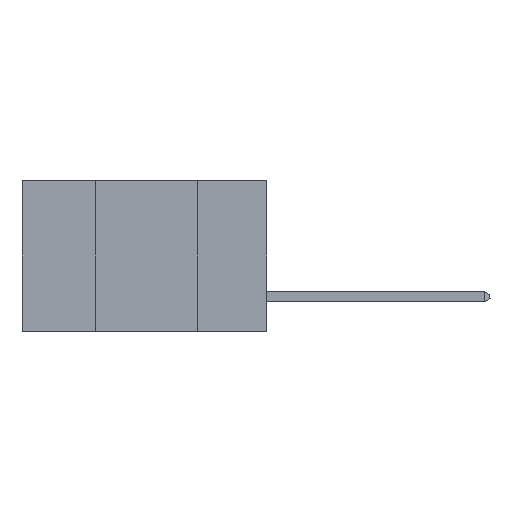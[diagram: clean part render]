
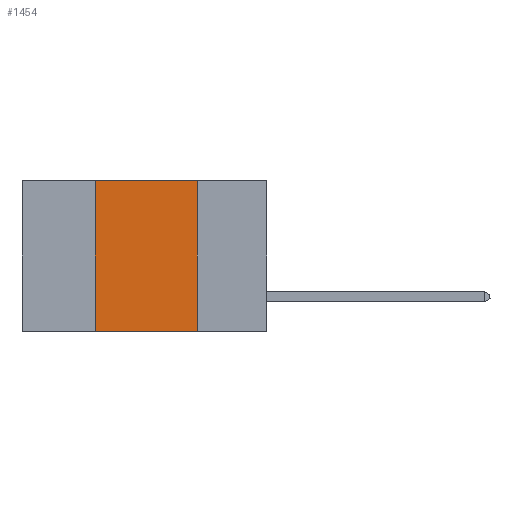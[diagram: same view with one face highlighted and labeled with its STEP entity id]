
A CAD part, left-side view. The second image highlights one B-rep face of the part: STEP entity #1454.
In plain terms, the highlighted planar face has unit normal (-1, 0, 0).
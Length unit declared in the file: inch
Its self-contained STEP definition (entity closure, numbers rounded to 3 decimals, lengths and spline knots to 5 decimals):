
#1454 = ADVANCED_FACE ( 'NONE', ( #32836 ), #9239, .F. ) ;
#3931 = LINE ( 'NONE', #7673, #34497 ) ;
#5997 = CARTESIAN_POINT ( 'NONE',  ( 0., 0.17, 0. ) ) ;
#7673 = CARTESIAN_POINT ( 'NONE',  ( 0., 0.42, 0. ) ) ;
#9239 = PLANE ( 'NONE',  #19675 ) ;
#11725 = VECTOR ( 'NONE', #15329, 39.37008 ) ;
#12020 = CARTESIAN_POINT ( 'NONE',  ( 0., 0.17, -0.37 ) ) ;
#12170 = VERTEX_POINT ( 'NONE', #34089 ) ;
#12734 = VERTEX_POINT ( 'NONE', #41839 ) ;
#12766 = ORIENTED_EDGE ( 'NONE', *, *, #40570, .T. ) ;
#13127 = CARTESIAN_POINT ( 'NONE',  ( 0., 0.6, -0.37 ) ) ;
#14165 = ORIENTED_EDGE ( 'NONE', *, *, #27347, .F. ) ;
#15329 = DIRECTION ( 'NONE',  ( 0., -1., 0. ) ) ;
#15983 = DIRECTION ( 'NONE',  ( 0., 0., -1. ) ) ;
#16390 = EDGE_CURVE ( 'NONE', #12734, #12170, #3931, .T. ) ;
#19675 = AXIS2_PLACEMENT_3D ( 'NONE', #21830, #28885, #15983 ) ;
#19760 = EDGE_LOOP ( 'NONE', ( #41641, #14165, #36043, #12766 ) ) ;
#20184 = VECTOR ( 'NONE', #40371, 39.37008 ) ;
#20535 = DIRECTION ( 'NONE',  ( 0., 0., 1. ) ) ;
#20976 = EDGE_CURVE ( 'NONE', #34721, #31734, #41512, .T. ) ;
#21830 = CARTESIAN_POINT ( 'NONE',  ( 0., 0.6, 0. ) ) ;
#27347 = EDGE_CURVE ( 'NONE', #12170, #34721, #34716, .T. ) ;
#28885 = DIRECTION ( 'NONE',  ( 1., 0., 0. ) ) ;
#29010 = LINE ( 'NONE', #13127, #11725 ) ;
#30162 = VECTOR ( 'NONE', #35528, 39.37008 ) ;
#30597 = CARTESIAN_POINT ( 'NONE',  ( 0., 0.17, 0. ) ) ;
#31734 = VERTEX_POINT ( 'NONE', #12020 ) ;
#32275 = CARTESIAN_POINT ( 'NONE',  ( 0., 0.6, 0. ) ) ;
#32836 = FACE_OUTER_BOUND ( 'NONE', #19760, .T. ) ;
#34089 = CARTESIAN_POINT ( 'NONE',  ( 0., 0.42, 0. ) ) ;
#34497 = VECTOR ( 'NONE', #20535, 39.37008 ) ;
#34716 = LINE ( 'NONE', #32275, #30162 ) ;
#34721 = VERTEX_POINT ( 'NONE', #5997 ) ;
#35528 = DIRECTION ( 'NONE',  ( 0., -1., 0. ) ) ;
#36043 = ORIENTED_EDGE ( 'NONE', *, *, #16390, .F. ) ;
#40371 = DIRECTION ( 'NONE',  ( 0., 0., -1. ) ) ;
#40570 = EDGE_CURVE ( 'NONE', #12734, #31734, #29010, .T. ) ;
#41512 = LINE ( 'NONE', #30597, #20184 ) ;
#41641 = ORIENTED_EDGE ( 'NONE', *, *, #20976, .F. ) ;
#41839 = CARTESIAN_POINT ( 'NONE',  ( 0., 0.42, -0.37 ) ) ;
